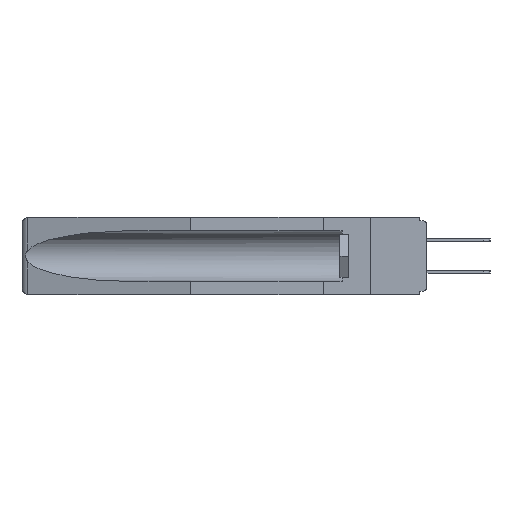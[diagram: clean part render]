
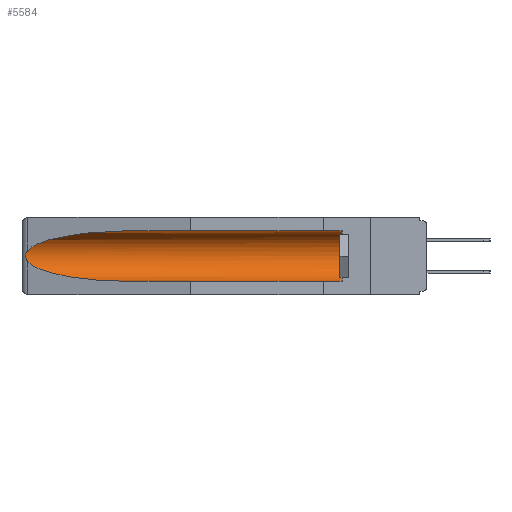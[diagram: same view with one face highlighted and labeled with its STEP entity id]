
A CAD part, left-side view. The second image highlights one B-rep face of the part: STEP entity #5584.
In plain terms, the highlighted cylindrical face has radius 2.857 mm (diameter 5.715 mm), a partial arc.
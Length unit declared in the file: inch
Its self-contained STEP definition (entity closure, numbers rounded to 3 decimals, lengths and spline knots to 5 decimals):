
#3 = VECTOR ( 'NONE', #11518, 39.37008 ) ;
#215 = CARTESIAN_POINT ( 'NONE',  ( 0.21114, 1.30732, -0.059 ) ) ;
#791 = ORIENTED_EDGE ( 'NONE', *, *, #14344, .T. ) ;
#1070 = ORIENTED_EDGE ( 'NONE', *, *, #14591, .F. ) ;
#1346 = VERTEX_POINT ( 'NONE', #19994 ) ;
#1491 = CARTESIAN_POINT ( 'NONE',  ( 0.26537, 1.52718, -0.19328 ) ) ;
#1554 = CARTESIAN_POINT ( 'NONE',  ( 0.155, -0.30754, -0.1715 ) ) ;
#1557 = DIRECTION ( 'NONE',  ( 0., 0., 1. ) ) ;
#1596 = CARTESIAN_POINT ( 'NONE',  ( 0.2673, 1.5327, -0.16383 ) ) ;
#1797 = CARTESIAN_POINT ( 'NONE',  ( 0.2673, 1.53269, -0.17917 ) ) ;
#3491 = DIRECTION ( 'NONE',  ( 0., -1., 0. ) ) ;
#5584 = ADVANCED_FACE ( 'NONE', ( #20976 ), #25481, .F. ) ;
#6789 = AXIS2_PLACEMENT_3D ( 'NONE', #1554, #17021, #12559 ) ;
#6812 = VERTEX_POINT ( 'NONE', #26467 ) ;
#7212 = CIRCLE ( 'NONE', #17538, 0.1125 ) ;
#8332 = CARTESIAN_POINT ( 'NONE',  ( 0.26654, 1.53092, -0.15636 ) ) ;
#8626 = ORIENTED_EDGE ( 'NONE', *, *, #11731, .T. ) ;
#9272 = ORIENTED_EDGE ( 'NONE', *, *, #25592, .T. ) ;
#11518 = DIRECTION ( 'NONE',  ( 0., 1., 0. ) ) ;
#11731 = EDGE_CURVE ( 'NONE', #6812, #19678, #27755, .T. ) ;
#11891 = B_SPLINE_CURVE_WITH_KNOTS ( 'NONE', 3,
 ( #14709, #21728, #8332, #1596, #19505, #19107, #1797, #19314, #23577, #1491 ),
 .UNSPECIFIED., .F., .F.,
 ( 4, 2, 2, 2, 4 ),
 ( 0., 0.00029, 0.00058, 0.00087, 0.00117 ),
 .UNSPECIFIED. ) ;
#12559 = DIRECTION ( 'NONE',  ( 0., 0., 1. ) ) ;
#12965 = CARTESIAN_POINT ( 'NONE',  ( 0.26537, 1.52718, -0.19328 ) ) ;
#13441 = EDGE_CURVE ( 'NONE', #23100, #1346, #7212, .T. ) ;
#14344 = EDGE_CURVE ( 'NONE', #19678, #26152, #11891, .T. ) ;
#14591 = EDGE_CURVE ( 'NONE', #23100, #24358, #23425, .T. ) ;
#14709 = CARTESIAN_POINT ( 'NONE',  ( 0.26537, 1.52718, -0.14972 ) ) ;
#15778 = CARTESIAN_POINT ( 'NONE',  ( 0.155, -0.30754, -0.059 ) ) ;
#16144 = CARTESIAN_POINT ( 'NONE',  ( 0.26537, 1.52718, -0.14972 ) ) ;
#16787 = DIRECTION ( 'NONE',  ( 0., 1., 0. ) ) ;
#16811 = VECTOR ( 'NONE', #16787, 39.37008 ) ;
#16996 = ORIENTED_EDGE ( 'NONE', *, *, #13441, .T. ) ;
#17021 = DIRECTION ( 'NONE',  ( 0., 1., 0. ) ) ;
#17129 = EDGE_LOOP ( 'NONE', ( #8626, #791, #9272, #1070, #16996, #26791 ) ) ;
#17538 = AXIS2_PLACEMENT_3D ( 'NONE', #27828, #3491, #1557 ) ;
#18110 = CARTESIAN_POINT ( 'NONE',  ( 0.155, 0.126, -0.284 ) ) ;
#18218 = CARTESIAN_POINT ( 'NONE',  ( 0.155, 1.07973, -0.284 ) ) ;
#18394 = CARTESIAN_POINT ( 'NONE',  ( 0.25451, 1.48313, -0.24835 ) ) ;
#19107 = CARTESIAN_POINT ( 'NONE',  ( 0.2675, 1.53308, -0.17534 ) ) ;
#19314 = CARTESIAN_POINT ( 'NONE',  ( 0.26655, 1.53094, -0.18657 ) ) ;
#19505 = CARTESIAN_POINT ( 'NONE',  ( 0.2675, 1.53308, -0.16763 ) ) ;
#19678 = VERTEX_POINT ( 'NONE', #16144 ) ;
#19994 = CARTESIAN_POINT ( 'NONE',  ( 0.155, 0.126, -0.059 ) ) ;
#20116 =( BOUNDED_CURVE ( )  B_SPLINE_CURVE ( 3, ( #20538, #18394, #20636, #18218 ),
 .UNSPECIFIED., .F., .F. ) 
 B_SPLINE_CURVE_WITH_KNOTS ( ( 4, 4 ),
 ( 0.1948, 1.5708 ),
 .UNSPECIFIED. ) 
 CURVE ( )  GEOMETRIC_REPRESENTATION_ITEM ( )  RATIONAL_B_SPLINE_CURVE ( ( 1., 0.848, 0.848, 1. ) ) 
 REPRESENTATION_ITEM ( '' )  );
#20277 = CARTESIAN_POINT ( 'NONE',  ( 0.26537, 1.52718, -0.14972 ) ) ;
#20538 = CARTESIAN_POINT ( 'NONE',  ( 0.26537, 1.52718, -0.19328 ) ) ;
#20636 = CARTESIAN_POINT ( 'NONE',  ( 0.21114, 1.30732, -0.284 ) ) ;
#20976 = FACE_OUTER_BOUND ( 'NONE', #17129, .T. ) ;
#21728 = CARTESIAN_POINT ( 'NONE',  ( 0.26597, 1.52961, -0.15275 ) ) ;
#21832 = LINE ( 'NONE', #15778, #3 ) ;
#23100 = VERTEX_POINT ( 'NONE', #18110 ) ;
#23304 = CARTESIAN_POINT ( 'NONE',  ( 0.155, -0.30754, -0.284 ) ) ;
#23425 = LINE ( 'NONE', #23304, #16811 ) ;
#23577 = CARTESIAN_POINT ( 'NONE',  ( 0.26597, 1.5296, -0.19026 ) ) ;
#24358 = VERTEX_POINT ( 'NONE', #26337 ) ;
#24639 = CARTESIAN_POINT ( 'NONE',  ( 0.25451, 1.48313, -0.09465 ) ) ;
#25481 = CYLINDRICAL_SURFACE ( 'NONE', #6789, 0.1125 ) ;
#25592 = EDGE_CURVE ( 'NONE', #26152, #24358, #20116, .T. ) ;
#26152 = VERTEX_POINT ( 'NONE', #12965 ) ;
#26337 = CARTESIAN_POINT ( 'NONE',  ( 0.155, 1.07973, -0.284 ) ) ;
#26467 = CARTESIAN_POINT ( 'NONE',  ( 0.155, 1.07973, -0.059 ) ) ;
#26604 = EDGE_CURVE ( 'NONE', #1346, #6812, #21832, .T. ) ;
#26690 = CARTESIAN_POINT ( 'NONE',  ( 0.155, 1.07973, -0.059 ) ) ;
#26791 = ORIENTED_EDGE ( 'NONE', *, *, #26604, .T. ) ;
#27755 =( BOUNDED_CURVE ( )  B_SPLINE_CURVE ( 3, ( #26690, #215, #24639, #20277 ),
 .UNSPECIFIED., .F., .F. ) 
 B_SPLINE_CURVE_WITH_KNOTS ( ( 4, 4 ),
 ( 4.71239, 6.08839 ),
 .UNSPECIFIED. ) 
 CURVE ( )  GEOMETRIC_REPRESENTATION_ITEM ( )  RATIONAL_B_SPLINE_CURVE ( ( 1., 0.848, 0.848, 1. ) ) 
 REPRESENTATION_ITEM ( '' )  );
#27828 = CARTESIAN_POINT ( 'NONE',  ( 0.155, 0.126, -0.1715 ) ) ;
